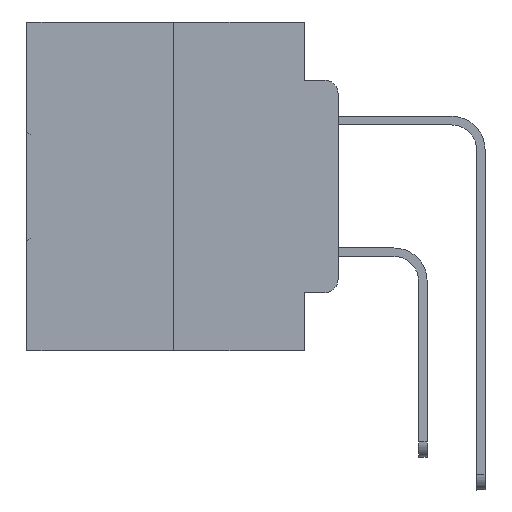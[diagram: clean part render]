
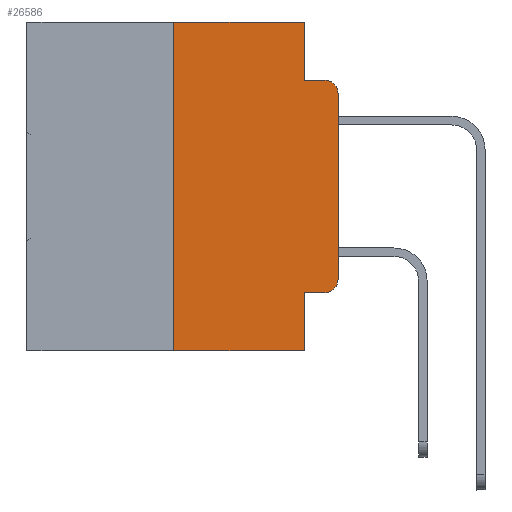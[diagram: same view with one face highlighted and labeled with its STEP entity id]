
A CAD part, left-side view. The second image highlights one B-rep face of the part: STEP entity #26586.
In plain terms, the highlighted planar face has unit normal (-1, 0, 0).
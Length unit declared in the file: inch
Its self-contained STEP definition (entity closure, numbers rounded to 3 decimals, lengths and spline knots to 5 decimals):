
#274 = DIRECTION ( 'NONE',  ( 0., 0., -1. ) ) ;
#305 = DIRECTION ( 'NONE',  ( -1., 0., 0. ) ) ;
#685 = AXIS2_PLACEMENT_3D ( 'NONE', #26867, #1299, #19293 ) ;
#740 = EDGE_CURVE ( 'NONE', #7855, #17717, #5757, .T. ) ;
#1299 = DIRECTION ( 'NONE',  ( 1., 0., 0. ) ) ;
#1637 = ORIENTED_EDGE ( 'NONE', *, *, #16362, .T. ) ;
#2680 = EDGE_CURVE ( 'NONE', #9270, #24549, #6841, .T. ) ;
#2981 = EDGE_CURVE ( 'NONE', #9773, #7855, #5249, .T. ) ;
#3141 = CARTESIAN_POINT ( 'NONE',  ( 0., 0.051, 0. ) ) ;
#3172 = CARTESIAN_POINT ( 'NONE',  ( 0., 0.25, 0. ) ) ;
#3208 = ORIENTED_EDGE ( 'NONE', *, *, #24032, .T. ) ;
#3529 = CARTESIAN_POINT ( 'NONE',  ( 0., 0.051, -0.4115 ) ) ;
#3777 = ORIENTED_EDGE ( 'NONE', *, *, #19607, .F. ) ;
#4338 = ORIENTED_EDGE ( 'NONE', *, *, #13062, .T. ) ;
#4592 = VECTOR ( 'NONE', #5782, 39.37008 ) ;
#4827 = ORIENTED_EDGE ( 'NONE', *, *, #2981, .T. ) ;
#4842 = CARTESIAN_POINT ( 'NONE',  ( 0., 0.473, -0.5 ) ) ;
#5249 = CIRCLE ( 'NONE', #15637, 0.02 ) ;
#5405 = LINE ( 'NONE', #3172, #4592 ) ;
#5603 = VECTOR ( 'NONE', #31499, 39.37008 ) ;
#5748 = DIRECTION ( 'NONE',  ( 0., 0., -1. ) ) ;
#5757 = LINE ( 'NONE', #26132, #13422 ) ;
#5782 = DIRECTION ( 'NONE',  ( 0., 0., 1. ) ) ;
#5834 = VECTOR ( 'NONE', #5748, 39.37008 ) ;
#6457 = LINE ( 'NONE', #9435, #20949 ) ;
#6667 = LINE ( 'NONE', #3141, #5834 ) ;
#6841 = LINE ( 'NONE', #22929, #26121 ) ;
#7463 = VERTEX_POINT ( 'NONE', #10326 ) ;
#7785 = VERTEX_POINT ( 'NONE', #11564 ) ;
#7855 = VERTEX_POINT ( 'NONE', #14326 ) ;
#7924 = EDGE_LOOP ( 'NONE', ( #29890, #4338, #25988, #19575, #26020, #30670, #3208, #3777, #1637, #4827 ) ) ;
#8611 = CARTESIAN_POINT ( 'NONE',  ( 0., 0.051, -0.0885 ) ) ;
#8777 = DIRECTION ( 'NONE',  ( 0., -1., 0. ) ) ;
#9270 = VERTEX_POINT ( 'NONE', #9785 ) ;
#9435 = CARTESIAN_POINT ( 'NONE',  ( 0., 0.473, 0. ) ) ;
#9773 = VERTEX_POINT ( 'NONE', #24519 ) ;
#9785 = CARTESIAN_POINT ( 'NONE',  ( 0., 0.051, 0. ) ) ;
#10326 = CARTESIAN_POINT ( 'NONE',  ( 0., 0.02, -0.0885 ) ) ;
#10469 = CARTESIAN_POINT ( 'NONE',  ( 0., 0.02, -0.1085 ) ) ;
#11194 = EDGE_CURVE ( 'NONE', #7785, #9270, #6457, .T. ) ;
#11386 = AXIS2_PLACEMENT_3D ( 'NONE', #10469, #28316, #13057 ) ;
#11564 = CARTESIAN_POINT ( 'NONE',  ( 0., 0.25, 0. ) ) ;
#12491 = LINE ( 'NONE', #8611, #5603 ) ;
#12646 = DIRECTION ( 'NONE',  ( 0., -1., 0. ) ) ;
#13057 = DIRECTION ( 'NONE',  ( 0., 0., -1. ) ) ;
#13062 = EDGE_CURVE ( 'NONE', #17717, #7463, #22785, .T. ) ;
#13113 = FACE_OUTER_BOUND ( 'NONE', #7924, .T. ) ;
#13422 = VECTOR ( 'NONE', #26172, 39.37008 ) ;
#14326 = CARTESIAN_POINT ( 'NONE',  ( 0., 0., -0.3915 ) ) ;
#15637 = AXIS2_PLACEMENT_3D ( 'NONE', #32217, #305, #274 ) ;
#16362 = EDGE_CURVE ( 'NONE', #25943, #9773, #24991, .T. ) ;
#16690 = CARTESIAN_POINT ( 'NONE',  ( 0., 0.25, -0.5 ) ) ;
#17086 = VERTEX_POINT ( 'NONE', #16690 ) ;
#17406 = VECTOR ( 'NONE', #8777, 39.37008 ) ;
#17717 = VERTEX_POINT ( 'NONE', #24456 ) ;
#19293 = DIRECTION ( 'NONE',  ( 0., 0., -1. ) ) ;
#19575 = ORIENTED_EDGE ( 'NONE', *, *, #2680, .F. ) ;
#19607 = EDGE_CURVE ( 'NONE', #25943, #26033, #6667, .T. ) ;
#20949 = VECTOR ( 'NONE', #27288, 39.37008 ) ;
#22471 = DIRECTION ( 'NONE',  ( 0., 0., -1. ) ) ;
#22785 = CIRCLE ( 'NONE', #11386, 0.02 ) ;
#22903 = LINE ( 'NONE', #4842, #29613 ) ;
#22929 = CARTESIAN_POINT ( 'NONE',  ( 0., 0.051, 0. ) ) ;
#24032 = EDGE_CURVE ( 'NONE', #17086, #26033, #22903, .T. ) ;
#24456 = CARTESIAN_POINT ( 'NONE',  ( 0., 0., -0.1085 ) ) ;
#24519 = CARTESIAN_POINT ( 'NONE',  ( 0., 0.02, -0.4115 ) ) ;
#24549 = VERTEX_POINT ( 'NONE', #31021 ) ;
#24991 = LINE ( 'NONE', #3529, #17406 ) ;
#25943 = VERTEX_POINT ( 'NONE', #29435 ) ;
#25988 = ORIENTED_EDGE ( 'NONE', *, *, #31134, .F. ) ;
#26020 = ORIENTED_EDGE ( 'NONE', *, *, #11194, .F. ) ;
#26033 = VERTEX_POINT ( 'NONE', #32241 ) ;
#26121 = VECTOR ( 'NONE', #22471, 39.37008 ) ;
#26132 = CARTESIAN_POINT ( 'NONE',  ( 0., 0., 0. ) ) ;
#26172 = DIRECTION ( 'NONE',  ( 0., 0., 1. ) ) ;
#26586 = ADVANCED_FACE ( 'NONE', ( #13113 ), #31875, .F. ) ;
#26867 = CARTESIAN_POINT ( 'NONE',  ( 0., 0.473, 0. ) ) ;
#27063 = EDGE_CURVE ( 'NONE', #17086, #7785, #5405, .T. ) ;
#27288 = DIRECTION ( 'NONE',  ( 0., -1., 0. ) ) ;
#28316 = DIRECTION ( 'NONE',  ( -1., 0., 0. ) ) ;
#29435 = CARTESIAN_POINT ( 'NONE',  ( 0., 0.051, -0.4115 ) ) ;
#29613 = VECTOR ( 'NONE', #12646, 39.37008 ) ;
#29890 = ORIENTED_EDGE ( 'NONE', *, *, #740, .T. ) ;
#30670 = ORIENTED_EDGE ( 'NONE', *, *, #27063, .F. ) ;
#31021 = CARTESIAN_POINT ( 'NONE',  ( 0., 0.051, -0.0885 ) ) ;
#31134 = EDGE_CURVE ( 'NONE', #24549, #7463, #12491, .T. ) ;
#31499 = DIRECTION ( 'NONE',  ( 0., -1., 0. ) ) ;
#31875 = PLANE ( 'NONE',  #685 ) ;
#32217 = CARTESIAN_POINT ( 'NONE',  ( 0., 0.02, -0.3915 ) ) ;
#32241 = CARTESIAN_POINT ( 'NONE',  ( 0., 0.051, -0.5 ) ) ;
